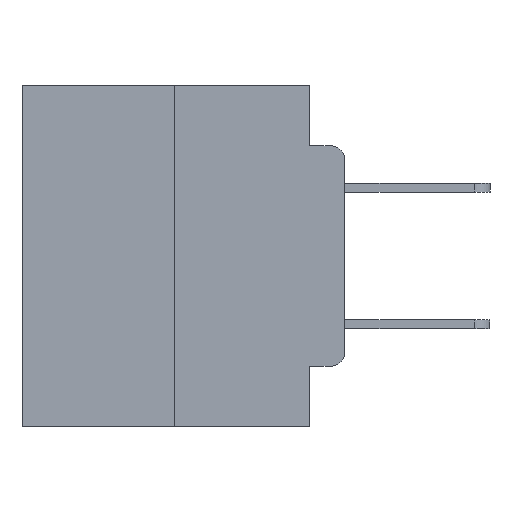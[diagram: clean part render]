
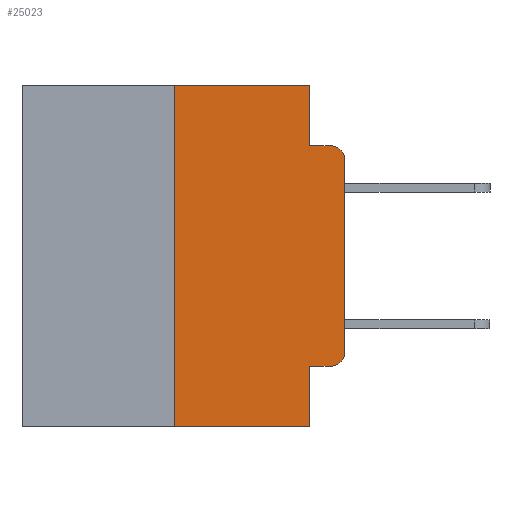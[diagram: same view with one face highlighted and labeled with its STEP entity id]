
A CAD part, left-side view. The second image highlights one B-rep face of the part: STEP entity #25023.
In plain terms, the highlighted planar face has unit normal (-1, 0, 0).
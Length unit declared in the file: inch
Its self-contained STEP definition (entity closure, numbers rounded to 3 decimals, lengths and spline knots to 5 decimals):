
#601 = VERTEX_POINT ( 'NONE', #10281 ) ;
#920 = VECTOR ( 'NONE', #22197, 39.37008 ) ;
#1120 = VERTEX_POINT ( 'NONE', #13797 ) ;
#1263 = EDGE_CURVE ( 'NONE', #13676, #16498, #26577, .T. ) ;
#1832 = CARTESIAN_POINT ( 'NONE',  ( 0., 0.02, -0.4115 ) ) ;
#2134 = DIRECTION ( 'NONE',  ( 0., -1., 0. ) ) ;
#2316 = DIRECTION ( 'NONE',  ( -1., 0., 0. ) ) ;
#2324 = CIRCLE ( 'NONE', #18624, 0.02 ) ;
#2899 = ORIENTED_EDGE ( 'NONE', *, *, #6725, .F. ) ;
#3596 = ORIENTED_EDGE ( 'NONE', *, *, #1263, .F. ) ;
#3939 = ORIENTED_EDGE ( 'NONE', *, *, #27265, .F. ) ;
#4073 = CIRCLE ( 'NONE', #23656, 0.02 ) ;
#4193 = LINE ( 'NONE', #20211, #20381 ) ;
#4359 = ORIENTED_EDGE ( 'NONE', *, *, #22892, .T. ) ;
#4916 = VERTEX_POINT ( 'NONE', #17697 ) ;
#5318 = LINE ( 'NONE', #17719, #27067 ) ;
#5387 = VERTEX_POINT ( 'NONE', #21563 ) ;
#5584 = EDGE_CURVE ( 'NONE', #23963, #16608, #17873, .T. ) ;
#6019 = ORIENTED_EDGE ( 'NONE', *, *, #8509, .T. ) ;
#6211 = CARTESIAN_POINT ( 'NONE',  ( 0., 0.473, 0. ) ) ;
#6725 = EDGE_CURVE ( 'NONE', #16498, #23963, #11842, .T. ) ;
#6836 = VECTOR ( 'NONE', #2134, 39.37008 ) ;
#7063 = CARTESIAN_POINT ( 'NONE',  ( 0., 0.02, -0.3915 ) ) ;
#7077 = EDGE_CURVE ( 'NONE', #16608, #601, #8824, .T. ) ;
#7206 = VERTEX_POINT ( 'NONE', #8255 ) ;
#7887 = CARTESIAN_POINT ( 'NONE',  ( 0., 0.051, -0.0885 ) ) ;
#8255 = CARTESIAN_POINT ( 'NONE',  ( 0., 0.051, -0.4115 ) ) ;
#8400 = DIRECTION ( 'NONE',  ( 0., 0., -1. ) ) ;
#8509 = EDGE_CURVE ( 'NONE', #5387, #601, #2324, .T. ) ;
#8824 = LINE ( 'NONE', #7887, #24898 ) ;
#8960 = VECTOR ( 'NONE', #12138, 39.37008 ) ;
#9197 = DIRECTION ( 'NONE',  ( 0., 0., -1. ) ) ;
#9773 = FACE_OUTER_BOUND ( 'NONE', #12467, .T. ) ;
#9891 = VECTOR ( 'NONE', #25513, 39.37008 ) ;
#10281 = CARTESIAN_POINT ( 'NONE',  ( 0., 0.02, -0.0885 ) ) ;
#10953 = ORIENTED_EDGE ( 'NONE', *, *, #11374, .T. ) ;
#11192 = VECTOR ( 'NONE', #23575, 39.37008 ) ;
#11374 = EDGE_CURVE ( 'NONE', #4916, #5387, #4193, .T. ) ;
#11842 = LINE ( 'NONE', #21430, #11192 ) ;
#12045 = CARTESIAN_POINT ( 'NONE',  ( 0., 0.051, 0. ) ) ;
#12138 = DIRECTION ( 'NONE',  ( 0., 0., -1. ) ) ;
#12467 = EDGE_LOOP ( 'NONE', ( #10953, #6019, #24118, #23782, #2899, #3596, #4359, #3939, #19433, #17022 ) ) ;
#12495 = LINE ( 'NONE', #23211, #6836 ) ;
#13676 = VERTEX_POINT ( 'NONE', #15126 ) ;
#13797 = CARTESIAN_POINT ( 'NONE',  ( 0., 0.051, -0.5 ) ) ;
#14581 = LINE ( 'NONE', #20375, #8960 ) ;
#15102 = CARTESIAN_POINT ( 'NONE',  ( 0., 0.02, -0.1085 ) ) ;
#15126 = CARTESIAN_POINT ( 'NONE',  ( 0., 0.25, -0.5 ) ) ;
#15823 = DIRECTION ( 'NONE',  ( 0., -1., 0. ) ) ;
#16498 = VERTEX_POINT ( 'NONE', #22936 ) ;
#16608 = VERTEX_POINT ( 'NONE', #19076 ) ;
#17022 = ORIENTED_EDGE ( 'NONE', *, *, #23054, .T. ) ;
#17206 = DIRECTION ( 'NONE',  ( 0., 0., -1. ) ) ;
#17697 = CARTESIAN_POINT ( 'NONE',  ( 0., 0., -0.3915 ) ) ;
#17719 = CARTESIAN_POINT ( 'NONE',  ( 0., 0.051, -0.4115 ) ) ;
#17873 = LINE ( 'NONE', #20083, #920 ) ;
#18151 = DIRECTION ( 'NONE',  ( 0., 0., 1. ) ) ;
#18624 = AXIS2_PLACEMENT_3D ( 'NONE', #15102, #2316, #17206 ) ;
#18822 = PLANE ( 'NONE',  #21872 ) ;
#19076 = CARTESIAN_POINT ( 'NONE',  ( 0., 0.051, -0.0885 ) ) ;
#19433 = ORIENTED_EDGE ( 'NONE', *, *, #25888, .T. ) ;
#20083 = CARTESIAN_POINT ( 'NONE',  ( 0., 0.051, 0. ) ) ;
#20211 = CARTESIAN_POINT ( 'NONE',  ( 0., 0., 0. ) ) ;
#20375 = CARTESIAN_POINT ( 'NONE',  ( 0., 0.051, 0. ) ) ;
#20381 = VECTOR ( 'NONE', #18151, 39.37008 ) ;
#20911 = DIRECTION ( 'NONE',  ( 1., 0., 0. ) ) ;
#21430 = CARTESIAN_POINT ( 'NONE',  ( 0., 0.473, 0. ) ) ;
#21563 = CARTESIAN_POINT ( 'NONE',  ( 0., 0., -0.1085 ) ) ;
#21711 = DIRECTION ( 'NONE',  ( -1., 0., 0. ) ) ;
#21872 = AXIS2_PLACEMENT_3D ( 'NONE', #6211, #20911, #8400 ) ;
#22197 = DIRECTION ( 'NONE',  ( 0., 0., -1. ) ) ;
#22892 = EDGE_CURVE ( 'NONE', #13676, #1120, #12495, .T. ) ;
#22936 = CARTESIAN_POINT ( 'NONE',  ( 0., 0.25, 0. ) ) ;
#23054 = EDGE_CURVE ( 'NONE', #23469, #4916, #4073, .T. ) ;
#23211 = CARTESIAN_POINT ( 'NONE',  ( 0., 0.473, -0.5 ) ) ;
#23469 = VERTEX_POINT ( 'NONE', #1832 ) ;
#23575 = DIRECTION ( 'NONE',  ( 0., -1., 0. ) ) ;
#23656 = AXIS2_PLACEMENT_3D ( 'NONE', #7063, #21711, #9197 ) ;
#23782 = ORIENTED_EDGE ( 'NONE', *, *, #5584, .F. ) ;
#23963 = VERTEX_POINT ( 'NONE', #12045 ) ;
#24118 = ORIENTED_EDGE ( 'NONE', *, *, #7077, .F. ) ;
#24898 = VECTOR ( 'NONE', #26664, 39.37008 ) ;
#25023 = ADVANCED_FACE ( 'NONE', ( #9773 ), #18822, .F. ) ;
#25513 = DIRECTION ( 'NONE',  ( 0., 0., 1. ) ) ;
#25888 = EDGE_CURVE ( 'NONE', #7206, #23469, #5318, .T. ) ;
#26379 = CARTESIAN_POINT ( 'NONE',  ( 0., 0.25, 0. ) ) ;
#26577 = LINE ( 'NONE', #26379, #9891 ) ;
#26664 = DIRECTION ( 'NONE',  ( 0., -1., 0. ) ) ;
#27067 = VECTOR ( 'NONE', #15823, 39.37008 ) ;
#27265 = EDGE_CURVE ( 'NONE', #7206, #1120, #14581, .T. ) ;
